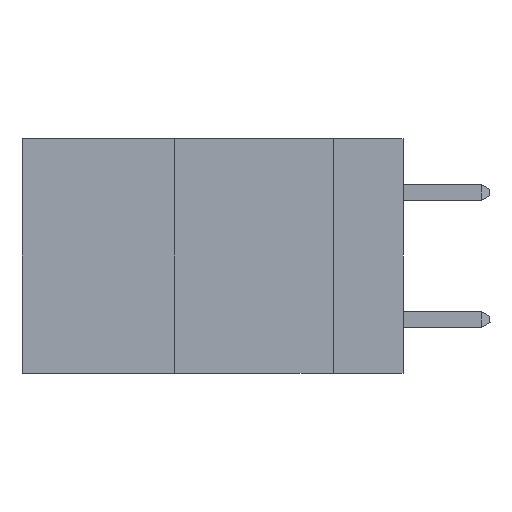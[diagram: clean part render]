
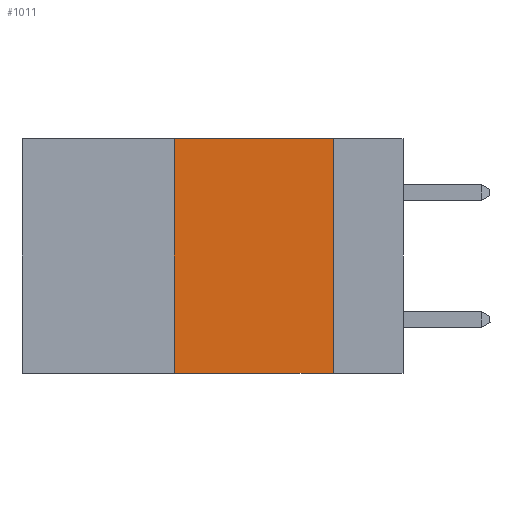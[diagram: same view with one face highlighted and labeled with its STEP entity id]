
A CAD part, left-side view. The second image highlights one B-rep face of the part: STEP entity #1011.
In plain terms, the highlighted planar face has unit normal (-1, 0, 0).
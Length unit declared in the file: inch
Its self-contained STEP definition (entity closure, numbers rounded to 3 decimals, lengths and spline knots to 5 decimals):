
#260 = FACE_OUTER_BOUND ( 'NONE', #861, .T. ) ;
#739 = VECTOR ( 'NONE', #3125, 39.37008 ) ;
#861 = EDGE_LOOP ( 'NONE', ( #4704, #9035, #8596, #5151 ) ) ;
#928 = LINE ( 'NONE', #2236, #4517 ) ;
#997 = VECTOR ( 'NONE', #6159, 39.37008 ) ;
#1011 = ADVANCED_FACE ( 'NONE', ( #260 ), #8474, .F. ) ;
#1411 = EDGE_CURVE ( 'NONE', #3282, #4175, #2218, .T. ) ;
#1493 = VECTOR ( 'NONE', #4724, 39.37008 ) ;
#1694 = VERTEX_POINT ( 'NONE', #9414 ) ;
#2124 = CARTESIAN_POINT ( 'NONE',  ( 0., 0.6, 0. ) ) ;
#2218 = LINE ( 'NONE', #8905, #739 ) ;
#2236 = CARTESIAN_POINT ( 'NONE',  ( 0., 0.11, 0. ) ) ;
#2468 = CARTESIAN_POINT ( 'NONE',  ( 0., 0.6, -0.37 ) ) ;
#3125 = DIRECTION ( 'NONE',  ( 0., 0., 1. ) ) ;
#3282 = VERTEX_POINT ( 'NONE', #8703 ) ;
#3628 = DIRECTION ( 'NONE',  ( 0., 0., -1. ) ) ;
#3720 = DIRECTION ( 'NONE',  ( 1., 0., 0. ) ) ;
#4175 = VERTEX_POINT ( 'NONE', #9598 ) ;
#4517 = VECTOR ( 'NONE', #6218, 39.37008 ) ;
#4704 = ORIENTED_EDGE ( 'NONE', *, *, #10053, .F. ) ;
#4724 = DIRECTION ( 'NONE',  ( 0., -1., 0. ) ) ;
#5151 = ORIENTED_EDGE ( 'NONE', *, *, #7121, .T. ) ;
#5394 = VERTEX_POINT ( 'NONE', #7854 ) ;
#5466 = LINE ( 'NONE', #10119, #997 ) ;
#6159 = DIRECTION ( 'NONE',  ( 0., -1., 0. ) ) ;
#6218 = DIRECTION ( 'NONE',  ( 0., 0., -1. ) ) ;
#6555 = EDGE_CURVE ( 'NONE', #4175, #1694, #5466, .T. ) ;
#7121 = EDGE_CURVE ( 'NONE', #3282, #5394, #8321, .T. ) ;
#7854 = CARTESIAN_POINT ( 'NONE',  ( 0., 0.11, -0.37 ) ) ;
#8321 = LINE ( 'NONE', #2468, #1493 ) ;
#8474 = PLANE ( 'NONE',  #9420 ) ;
#8596 = ORIENTED_EDGE ( 'NONE', *, *, #1411, .F. ) ;
#8703 = CARTESIAN_POINT ( 'NONE',  ( 0., 0.36, -0.37 ) ) ;
#8905 = CARTESIAN_POINT ( 'NONE',  ( 0., 0.36, 0. ) ) ;
#9035 = ORIENTED_EDGE ( 'NONE', *, *, #6555, .F. ) ;
#9414 = CARTESIAN_POINT ( 'NONE',  ( 0., 0.11, 0. ) ) ;
#9420 = AXIS2_PLACEMENT_3D ( 'NONE', #2124, #3720, #3628 ) ;
#9598 = CARTESIAN_POINT ( 'NONE',  ( 0., 0.36, 0. ) ) ;
#10053 = EDGE_CURVE ( 'NONE', #1694, #5394, #928, .T. ) ;
#10119 = CARTESIAN_POINT ( 'NONE',  ( 0., 0.6, 0. ) ) ;
